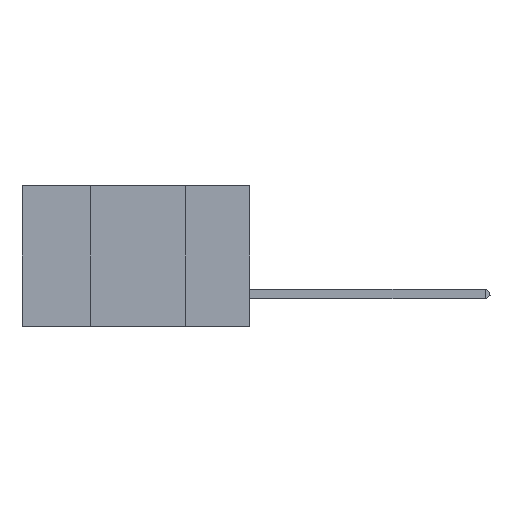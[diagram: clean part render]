
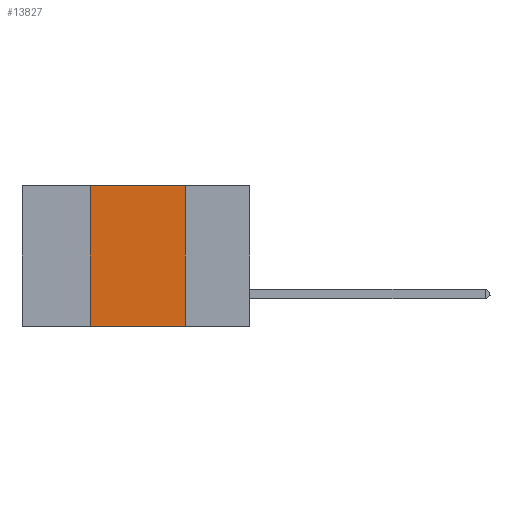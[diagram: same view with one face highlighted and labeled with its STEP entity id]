
A CAD part, left-side view. The second image highlights one B-rep face of the part: STEP entity #13827.
In plain terms, the highlighted planar face has unit normal (-1, 0, 0).
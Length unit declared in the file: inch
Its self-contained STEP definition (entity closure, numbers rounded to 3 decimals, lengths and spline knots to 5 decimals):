
#274 = LINE ( 'NONE', #5554, #6931 ) ;
#545 = PLANE ( 'NONE',  #11275 ) ;
#777 = DIRECTION ( 'NONE',  ( 0., 0., -1. ) ) ;
#1918 = EDGE_CURVE ( 'NONE', #19813, #20773, #15873, .T. ) ;
#2861 = DIRECTION ( 'NONE',  ( 0., -1., 0. ) ) ;
#5551 = DIRECTION ( 'NONE',  ( 1., 0., 0. ) ) ;
#5554 = CARTESIAN_POINT ( 'NONE',  ( 0., 0.6, 0. ) ) ;
#5801 = ORIENTED_EDGE ( 'NONE', *, *, #1918, .T. ) ;
#6110 = ORIENTED_EDGE ( 'NONE', *, *, #7105, .F. ) ;
#6234 = CARTESIAN_POINT ( 'NONE',  ( 0., 0.42, 0. ) ) ;
#6604 = EDGE_LOOP ( 'NONE', ( #8448, #8735, #6110, #5801 ) ) ;
#6883 = CARTESIAN_POINT ( 'NONE',  ( 0., 0.17, -0.37 ) ) ;
#6931 = VECTOR ( 'NONE', #17264, 39.37008 ) ;
#7105 = EDGE_CURVE ( 'NONE', #19813, #18131, #13795, .T. ) ;
#7213 = CARTESIAN_POINT ( 'NONE',  ( 0., 0.42, -0.37 ) ) ;
#8448 = ORIENTED_EDGE ( 'NONE', *, *, #10659, .F. ) ;
#8735 = ORIENTED_EDGE ( 'NONE', *, *, #15613, .F. ) ;
#9001 = LINE ( 'NONE', #20414, #9282 ) ;
#9282 = VECTOR ( 'NONE', #777, 39.37008 ) ;
#9593 = DIRECTION ( 'NONE',  ( 0., 0., 1. ) ) ;
#9675 = VECTOR ( 'NONE', #9593, 39.37008 ) ;
#10659 = EDGE_CURVE ( 'NONE', #13772, #20773, #9001, .T. ) ;
#11275 = AXIS2_PLACEMENT_3D ( 'NONE', #11862, #5551, #17117 ) ;
#11626 = CARTESIAN_POINT ( 'NONE',  ( 0., 0.6, -0.37 ) ) ;
#11686 = VECTOR ( 'NONE', #2861, 39.37008 ) ;
#11862 = CARTESIAN_POINT ( 'NONE',  ( 0., 0.6, 0. ) ) ;
#13514 = CARTESIAN_POINT ( 'NONE',  ( 0., 0.17, 0. ) ) ;
#13553 = CARTESIAN_POINT ( 'NONE',  ( 0., 0.42, 0. ) ) ;
#13772 = VERTEX_POINT ( 'NONE', #13514 ) ;
#13795 = LINE ( 'NONE', #6234, #9675 ) ;
#13827 = ADVANCED_FACE ( 'NONE', ( #19848 ), #545, .F. ) ;
#15613 = EDGE_CURVE ( 'NONE', #18131, #13772, #274, .T. ) ;
#15873 = LINE ( 'NONE', #11626, #11686 ) ;
#17117 = DIRECTION ( 'NONE',  ( 0., 0., -1. ) ) ;
#17264 = DIRECTION ( 'NONE',  ( 0., -1., 0. ) ) ;
#18131 = VERTEX_POINT ( 'NONE', #13553 ) ;
#19813 = VERTEX_POINT ( 'NONE', #7213 ) ;
#19848 = FACE_OUTER_BOUND ( 'NONE', #6604, .T. ) ;
#20414 = CARTESIAN_POINT ( 'NONE',  ( 0., 0.17, 0. ) ) ;
#20773 = VERTEX_POINT ( 'NONE', #6883 ) ;
